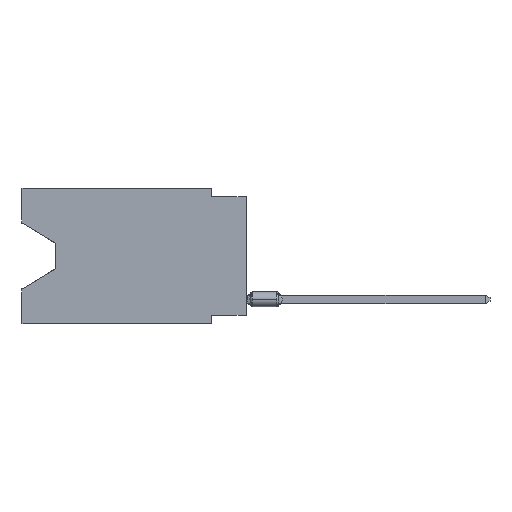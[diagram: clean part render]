
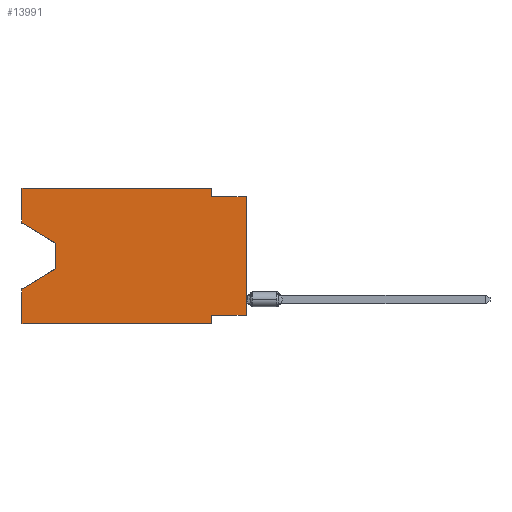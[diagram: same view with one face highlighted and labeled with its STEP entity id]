
A CAD part, left-side view. The second image highlights one B-rep face of the part: STEP entity #13991.
In plain terms, the highlighted planar face has unit normal (-1, 0, 0).
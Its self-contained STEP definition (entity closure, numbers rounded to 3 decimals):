
#168 = VERTEX_POINT ( 'NONE', #3009 ) ;
#293 = CARTESIAN_POINT ( 'NONE',  ( 0., 2.54, -9.271 ) ) ;
#786 = ORIENTED_EDGE ( 'NONE', *, *, #9513, .F. ) ;
#977 = LINE ( 'NONE', #17490, #15869 ) ;
#1334 = VERTEX_POINT ( 'NONE', #18469 ) ;
#1366 = EDGE_CURVE ( 'NONE', #1334, #18660, #2085, .T. ) ;
#1416 = VERTEX_POINT ( 'NONE', #14497 ) ;
#1477 = EDGE_CURVE ( 'NONE', #13199, #168, #977, .T. ) ;
#1574 = DIRECTION ( 'NONE',  ( 0., 0., -1. ) ) ;
#1620 = ORIENTED_EDGE ( 'NONE', *, *, #1366, .F. ) ;
#1957 = EDGE_CURVE ( 'NONE', #1334, #16163, #11955, .T. ) ;
#2085 = LINE ( 'NONE', #8233, #12996 ) ;
#2210 = DIRECTION ( 'NONE',  ( 0., -0.855, -0.519 ) ) ;
#2236 = ORIENTED_EDGE ( 'NONE', *, *, #10228, .F. ) ;
#2289 = CARTESIAN_POINT ( 'NONE',  ( 0., 16.383, 0. ) ) ;
#2352 = VECTOR ( 'NONE', #6420, 1000. ) ;
#3009 = CARTESIAN_POINT ( 'NONE',  ( 0., 13.97, -5.893 ) ) ;
#3815 = EDGE_CURVE ( 'NONE', #15879, #10008, #11460, .T. ) ;
#3818 = LINE ( 'NONE', #18609, #11257 ) ;
#3926 = LINE ( 'NONE', #10055, #5485 ) ;
#4099 = ORIENTED_EDGE ( 'NONE', *, *, #17776, .T. ) ;
#4641 = CARTESIAN_POINT ( 'NONE',  ( 0., 16.383, -9.906 ) ) ;
#4685 = CARTESIAN_POINT ( 'NONE',  ( 0., 16.383, 0. ) ) ;
#4739 = EDGE_CURVE ( 'NONE', #15879, #13199, #3818, .T. ) ;
#4794 = DIRECTION ( 'NONE',  ( 0., 0., -1. ) ) ;
#4975 = LINE ( 'NONE', #6454, #17819 ) ;
#5071 = DIRECTION ( 'NONE',  ( 0., 0.855, -0.519 ) ) ;
#5469 = AXIS2_PLACEMENT_3D ( 'NONE', #4685, #15196, #1574 ) ;
#5485 = VECTOR ( 'NONE', #18706, 1000. ) ;
#6420 = DIRECTION ( 'NONE',  ( 0., -1., 0. ) ) ;
#6454 = CARTESIAN_POINT ( 'NONE',  ( 0., 13.97, -5.893 ) ) ;
#6869 = CARTESIAN_POINT ( 'NONE',  ( 0., 16.383, 0. ) ) ;
#7106 = CARTESIAN_POINT ( 'NONE',  ( 0., 16.383, 0. ) ) ;
#7241 = CARTESIAN_POINT ( 'NONE',  ( 0., 2.54, 0. ) ) ;
#7652 = PLANE ( 'NONE',  #5469 ) ;
#7954 = CARTESIAN_POINT ( 'NONE',  ( 0., 2.54, -9.906 ) ) ;
#8233 = CARTESIAN_POINT ( 'NONE',  ( 0., 0., -9.271 ) ) ;
#8283 = DIRECTION ( 'NONE',  ( 0., 0., 1. ) ) ;
#8531 = DIRECTION ( 'NONE',  ( 0., 0., -1. ) ) ;
#8560 = ORIENTED_EDGE ( 'NONE', *, *, #14240, .F. ) ;
#8616 = EDGE_CURVE ( 'NONE', #168, #1416, #4975, .T. ) ;
#8639 = CARTESIAN_POINT ( 'NONE',  ( 0., 0., -0.635 ) ) ;
#8799 = DIRECTION ( 'NONE',  ( 0., 0., 1. ) ) ;
#8981 = CARTESIAN_POINT ( 'NONE',  ( 0., 2.54, -0.635 ) ) ;
#9513 = EDGE_CURVE ( 'NONE', #13022, #1416, #3926, .T. ) ;
#9527 = DIRECTION ( 'NONE',  ( 0., 1., 0. ) ) ;
#9822 = LINE ( 'NONE', #6869, #10479 ) ;
#9828 = VERTEX_POINT ( 'NONE', #12108 ) ;
#10008 = VERTEX_POINT ( 'NONE', #2289 ) ;
#10055 = CARTESIAN_POINT ( 'NONE',  ( 0., 16.383, 0. ) ) ;
#10222 = ORIENTED_EDGE ( 'NONE', *, *, #1957, .T. ) ;
#10228 = EDGE_CURVE ( 'NONE', #11675, #16163, #17503, .T. ) ;
#10314 = CARTESIAN_POINT ( 'NONE',  ( 0., 13.97, -4.013 ) ) ;
#10479 = VECTOR ( 'NONE', #13097, 1000. ) ;
#10930 = ORIENTED_EDGE ( 'NONE', *, *, #3815, .F. ) ;
#11097 = ORIENTED_EDGE ( 'NONE', *, *, #1477, .T. ) ;
#11105 = EDGE_CURVE ( 'NONE', #10008, #16955, #9822, .T. ) ;
#11257 = VECTOR ( 'NONE', #2210, 1000. ) ;
#11410 = CARTESIAN_POINT ( 'NONE',  ( 0., 16.383, -9.906 ) ) ;
#11460 = LINE ( 'NONE', #7106, #16309 ) ;
#11675 = VERTEX_POINT ( 'NONE', #8981 ) ;
#11955 = LINE ( 'NONE', #14943, #13638 ) ;
#12108 = CARTESIAN_POINT ( 'NONE',  ( 0., 2.54, -9.906 ) ) ;
#12208 = FACE_OUTER_BOUND ( 'NONE', #14147, .T. ) ;
#12311 = LINE ( 'NONE', #7954, #14661 ) ;
#12996 = VECTOR ( 'NONE', #9527, 1000. ) ;
#13022 = VERTEX_POINT ( 'NONE', #11410 ) ;
#13050 = DIRECTION ( 'NONE',  ( 0., 0., -1. ) ) ;
#13097 = DIRECTION ( 'NONE',  ( 0., -1., 0. ) ) ;
#13199 = VERTEX_POINT ( 'NONE', #10314 ) ;
#13339 = VECTOR ( 'NONE', #14600, 1000. ) ;
#13425 = ORIENTED_EDGE ( 'NONE', *, *, #11105, .F. ) ;
#13638 = VECTOR ( 'NONE', #8799, 1000. ) ;
#13945 = LINE ( 'NONE', #4641, #2352 ) ;
#13962 = EDGE_CURVE ( 'NONE', #16955, #11675, #16764, .T. ) ;
#13991 = ADVANCED_FACE ( 'NONE', ( #12208 ), #7652, .F. ) ;
#14147 = EDGE_LOOP ( 'NONE', ( #14157, #11097, #17942, #786, #4099, #8560, #1620, #10222, #2236, #17671, #13425, #10930 ) ) ;
#14157 = ORIENTED_EDGE ( 'NONE', *, *, #4739, .T. ) ;
#14240 = EDGE_CURVE ( 'NONE', #18660, #9828, #12311, .T. ) ;
#14497 = CARTESIAN_POINT ( 'NONE',  ( 0., 16.383, -7.36 ) ) ;
#14600 = DIRECTION ( 'NONE',  ( 0., -1., 0. ) ) ;
#14661 = VECTOR ( 'NONE', #4794, 1000. ) ;
#14943 = CARTESIAN_POINT ( 'NONE',  ( 0., 0., 0. ) ) ;
#14970 = VECTOR ( 'NONE', #13050, 1000. ) ;
#15196 = DIRECTION ( 'NONE',  ( 1., 0., 0. ) ) ;
#15869 = VECTOR ( 'NONE', #8531, 1000. ) ;
#15879 = VERTEX_POINT ( 'NONE', #19012 ) ;
#16163 = VERTEX_POINT ( 'NONE', #16412 ) ;
#16309 = VECTOR ( 'NONE', #8283, 1000. ) ;
#16412 = CARTESIAN_POINT ( 'NONE',  ( 0., 0., -0.635 ) ) ;
#16764 = LINE ( 'NONE', #18185, #14970 ) ;
#16955 = VERTEX_POINT ( 'NONE', #7241 ) ;
#17490 = CARTESIAN_POINT ( 'NONE',  ( 0., 13.97, -4.013 ) ) ;
#17503 = LINE ( 'NONE', #8639, #13339 ) ;
#17671 = ORIENTED_EDGE ( 'NONE', *, *, #13962, .F. ) ;
#17776 = EDGE_CURVE ( 'NONE', #13022, #9828, #13945, .T. ) ;
#17819 = VECTOR ( 'NONE', #5071, 1000. ) ;
#17942 = ORIENTED_EDGE ( 'NONE', *, *, #8616, .T. ) ;
#18185 = CARTESIAN_POINT ( 'NONE',  ( 0., 2.54, 0. ) ) ;
#18469 = CARTESIAN_POINT ( 'NONE',  ( 0., 0., -9.271 ) ) ;
#18609 = CARTESIAN_POINT ( 'NONE',  ( 0., 16.383, -2.546 ) ) ;
#18660 = VERTEX_POINT ( 'NONE', #293 ) ;
#18706 = DIRECTION ( 'NONE',  ( 0., 0., 1. ) ) ;
#19012 = CARTESIAN_POINT ( 'NONE',  ( 0., 16.383, -2.546 ) ) ;
